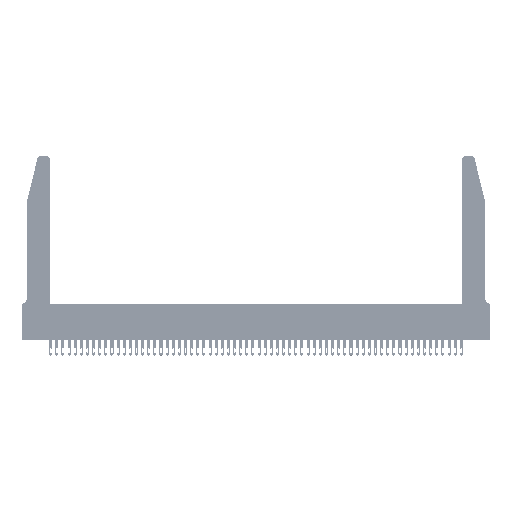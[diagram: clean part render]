
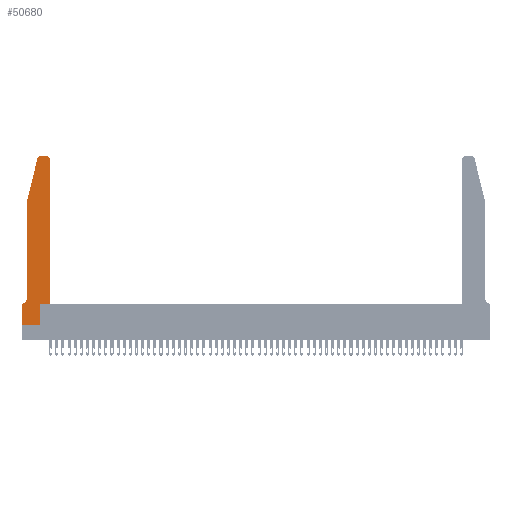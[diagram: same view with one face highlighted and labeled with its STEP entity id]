
A CAD part, top view. The second image highlights one B-rep face of the part: STEP entity #50680.
In plain terms, the highlighted planar face has unit normal (0, 0, 1).
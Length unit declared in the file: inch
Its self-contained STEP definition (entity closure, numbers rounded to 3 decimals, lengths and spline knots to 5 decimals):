
#608 = DIRECTION ( 'NONE',  ( 1., 0., 0. ) ) ;
#751 = ORIENTED_EDGE ( 'NONE', *, *, #6503, .T. ) ;
#1708 = CARTESIAN_POINT ( 'NONE',  ( 0.4505, 2.72, 0.37 ) ) ;
#1716 = VERTEX_POINT ( 'NONE', #50144 ) ;
#2566 = LINE ( 'NONE', #47520, #11103 ) ;
#3043 = EDGE_CURVE ( 'NONE', #32158, #43014, #36779, .T. ) ;
#3325 = VECTOR ( 'NONE', #35765, 39.37008 ) ;
#3349 = AXIS2_PLACEMENT_3D ( 'NONE', #44101, #18902, #6408 ) ;
#3916 = EDGE_CURVE ( 'NONE', #26741, #7432, #30757, .T. ) ;
#4082 = CARTESIAN_POINT ( 'NONE',  ( 0.0055, 0.35, 0.37 ) ) ;
#4128 = ORIENTED_EDGE ( 'NONE', *, *, #3043, .T. ) ;
#4627 = LINE ( 'NONE', #18191, #50087 ) ;
#5911 = CARTESIAN_POINT ( 'NONE',  ( 0.284, 2.72, 0.37 ) ) ;
#6408 = DIRECTION ( 'NONE',  ( 1., 0., 0. ) ) ;
#6444 = DIRECTION ( 'NONE',  ( 1., 0., 0. ) ) ;
#6503 = EDGE_CURVE ( 'NONE', #1716, #32158, #38301, .T. ) ;
#6535 = ORIENTED_EDGE ( 'NONE', *, *, #54169, .T. ) ;
#7432 = VERTEX_POINT ( 'NONE', #36274 ) ;
#7606 = AXIS2_PLACEMENT_3D ( 'NONE', #5911, #23523, #6444 ) ;
#7684 = CARTESIAN_POINT ( 'NONE',  ( 0.4205, 2.75, 0.37 ) ) ;
#9688 = VECTOR ( 'NONE', #32460, 39.37008 ) ;
#11103 = VECTOR ( 'NONE', #30759, 39.37008 ) ;
#11138 = CARTESIAN_POINT ( 'NONE',  ( 0.4505, 0.35, 0.37 ) ) ;
#11322 = CARTESIAN_POINT ( 'NONE',  ( 0.0755, 2., 0.37 ) ) ;
#12737 = DIRECTION ( 'NONE',  ( 1., 0., 0. ) ) ;
#12783 = CARTESIAN_POINT ( 'NONE',  ( 0.0755, 0.35, 0.37 ) ) ;
#13204 = CARTESIAN_POINT ( 'NONE',  ( 0., 0., 0.37 ) ) ;
#15242 = EDGE_CURVE ( 'NONE', #44649, #21769, #23049, .T. ) ;
#15434 = EDGE_CURVE ( 'NONE', #7432, #22661, #4627, .T. ) ;
#16337 = VERTEX_POINT ( 'NONE', #31520 ) ;
#16687 = AXIS2_PLACEMENT_3D ( 'NONE', #39006, #21898, #608 ) ;
#18191 = CARTESIAN_POINT ( 'NONE',  ( 0.0755, 2., 0.37 ) ) ;
#18579 = EDGE_CURVE ( 'NONE', #43014, #40114, #18795, .T. ) ;
#18660 = CARTESIAN_POINT ( 'NONE',  ( 0.2605, 2.75, 0.37 ) ) ;
#18795 = CIRCLE ( 'NONE', #16687, 0.03 ) ;
#18902 = DIRECTION ( 'NONE',  ( 0., 0., 1. ) ) ;
#19338 = DIRECTION ( 'NONE',  ( 0., 0., -1. ) ) ;
#21769 = VERTEX_POINT ( 'NONE', #33777 ) ;
#21898 = DIRECTION ( 'NONE',  ( 0., 0., 1. ) ) ;
#22661 = VERTEX_POINT ( 'NONE', #44917 ) ;
#23049 = LINE ( 'NONE', #13204, #30980 ) ;
#23162 = VERTEX_POINT ( 'NONE', #38776 ) ;
#23523 = DIRECTION ( 'NONE',  ( 0., 0., 1. ) ) ;
#24014 = ORIENTED_EDGE ( 'NONE', *, *, #15242, .T. ) ;
#24018 = FACE_OUTER_BOUND ( 'NONE', #33427, .T. ) ;
#24447 = VECTOR ( 'NONE', #46647, 39.37008 ) ;
#25323 = ORIENTED_EDGE ( 'NONE', *, *, #3916, .T. ) ;
#25496 = CARTESIAN_POINT ( 'NONE',  ( 0.4505, 0.35, 0.37 ) ) ;
#25924 = ORIENTED_EDGE ( 'NONE', *, *, #15434, .T. ) ;
#26399 = VERTEX_POINT ( 'NONE', #4082 ) ;
#26741 = VERTEX_POINT ( 'NONE', #36958 ) ;
#27054 = ORIENTED_EDGE ( 'NONE', *, *, #42990, .T. ) ;
#30408 = LINE ( 'NONE', #33695, #50222 ) ;
#30757 = LINE ( 'NONE', #11322, #9688 ) ;
#30759 = DIRECTION ( 'NONE',  ( 0., 1., 0. ) ) ;
#30980 = VECTOR ( 'NONE', #34140, 39.37008 ) ;
#31052 = DIRECTION ( 'NONE',  ( 0., -1., 0. ) ) ;
#31520 = CARTESIAN_POINT ( 'NONE',  ( 0.2865, 0., 0.37 ) ) ;
#31794 = EDGE_CURVE ( 'NONE', #23162, #26741, #45895, .T. ) ;
#31848 = CARTESIAN_POINT ( 'NONE',  ( 0.0055, 0.42, 0.37 ) ) ;
#32158 = VERTEX_POINT ( 'NONE', #25496 ) ;
#32280 = LINE ( 'NONE', #18660, #3325 ) ;
#32460 = DIRECTION ( 'NONE',  ( -0.239, -0.971, 0. ) ) ;
#33427 = EDGE_LOOP ( 'NONE', ( #6535, #52110, #25323, #25924, #52306, #34931, #24014, #44092, #27054, #751, #4128, #45435 ) ) ;
#33695 = CARTESIAN_POINT ( 'NONE',  ( 0., 0., 0.37 ) ) ;
#33771 = CARTESIAN_POINT ( 'NONE',  ( 0.4505, 0.35, 0.37 ) ) ;
#33777 = CARTESIAN_POINT ( 'NONE',  ( 0., 0., 0.37 ) ) ;
#33861 = EDGE_CURVE ( 'NONE', #26399, #44649, #51608, .T. ) ;
#34140 = DIRECTION ( 'NONE',  ( 0., -1., 0. ) ) ;
#34931 = ORIENTED_EDGE ( 'NONE', *, *, #33861, .T. ) ;
#35765 = DIRECTION ( 'NONE',  ( -1., 0., 0. ) ) ;
#35834 = CARTESIAN_POINT ( 'NONE',  ( 0., 0.35, 0.37 ) ) ;
#36274 = CARTESIAN_POINT ( 'NONE',  ( 0.0755, 2., 0.37 ) ) ;
#36523 = DIRECTION ( 'NONE',  ( 0., 1., 0. ) ) ;
#36779 = LINE ( 'NONE', #11138, #45986 ) ;
#36958 = CARTESIAN_POINT ( 'NONE',  ( 0.25487, 2.72718, 0.37 ) ) ;
#38301 = LINE ( 'NONE', #33771, #24447 ) ;
#38776 = CARTESIAN_POINT ( 'NONE',  ( 0.284, 2.75, 0.37 ) ) ;
#38841 = AXIS2_PLACEMENT_3D ( 'NONE', #31848, #19338, #40128 ) ;
#38932 = CIRCLE ( 'NONE', #38841, 0.07 ) ;
#39006 = CARTESIAN_POINT ( 'NONE',  ( 0.4205, 2.72, 0.37 ) ) ;
#40114 = VERTEX_POINT ( 'NONE', #7684 ) ;
#40128 = DIRECTION ( 'NONE',  ( -1., 0., 0. ) ) ;
#40884 = EDGE_CURVE ( 'NONE', #21769, #16337, #30408, .T. ) ;
#42990 = EDGE_CURVE ( 'NONE', #16337, #1716, #2566, .T. ) ;
#43002 = VECTOR ( 'NONE', #50373, 39.37008 ) ;
#43014 = VERTEX_POINT ( 'NONE', #1708 ) ;
#44092 = ORIENTED_EDGE ( 'NONE', *, *, #40884, .T. ) ;
#44101 = CARTESIAN_POINT ( 'NONE',  ( 0., 0.35, 0.37 ) ) ;
#44649 = VERTEX_POINT ( 'NONE', #35834 ) ;
#44917 = CARTESIAN_POINT ( 'NONE',  ( 0.0755, 0.42, 0.37 ) ) ;
#45435 = ORIENTED_EDGE ( 'NONE', *, *, #18579, .T. ) ;
#45895 = CIRCLE ( 'NONE', #7606, 0.03 ) ;
#45986 = VECTOR ( 'NONE', #36523, 39.37008 ) ;
#46647 = DIRECTION ( 'NONE',  ( 1., 0., 0. ) ) ;
#47291 = EDGE_CURVE ( 'NONE', #22661, #26399, #38932, .T. ) ;
#47520 = CARTESIAN_POINT ( 'NONE',  ( 0.2865, 0.35, 0.37 ) ) ;
#48164 = PLANE ( 'NONE',  #3349 ) ;
#50087 = VECTOR ( 'NONE', #31052, 39.37008 ) ;
#50144 = CARTESIAN_POINT ( 'NONE',  ( 0.2865, 0.35, 0.37 ) ) ;
#50222 = VECTOR ( 'NONE', #12737, 39.37008 ) ;
#50373 = DIRECTION ( 'NONE',  ( -1., 0., 0. ) ) ;
#50680 = ADVANCED_FACE ( 'NONE', ( #24018 ), #48164, .T. ) ;
#51608 = LINE ( 'NONE', #12783, #43002 ) ;
#52110 = ORIENTED_EDGE ( 'NONE', *, *, #31794, .T. ) ;
#52306 = ORIENTED_EDGE ( 'NONE', *, *, #47291, .T. ) ;
#54169 = EDGE_CURVE ( 'NONE', #40114, #23162, #32280, .T. ) ;
